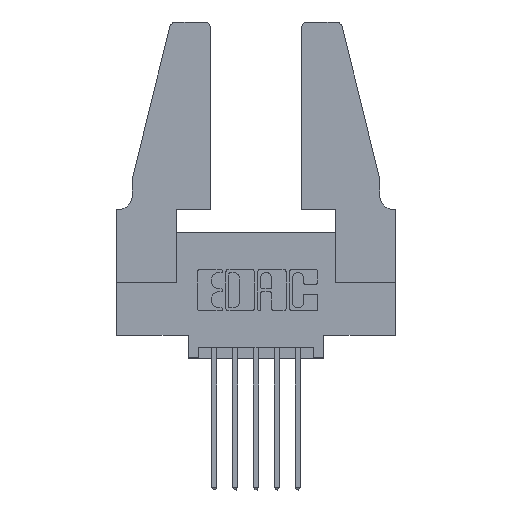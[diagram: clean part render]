
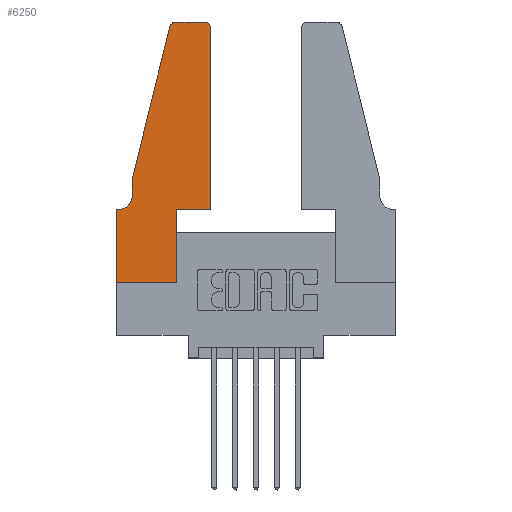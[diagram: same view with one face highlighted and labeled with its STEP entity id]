
A CAD part, top view. The second image highlights one B-rep face of the part: STEP entity #6250.
In plain terms, the highlighted planar face has unit normal (0, 0, 1).
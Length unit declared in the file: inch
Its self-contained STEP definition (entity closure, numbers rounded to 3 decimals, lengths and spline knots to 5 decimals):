
#84 = VERTEX_POINT ( 'NONE', #4923 ) ;
#313 = AXIS2_PLACEMENT_3D ( 'NONE', #5405, #5387, #5365 ) ;
#339 = VERTEX_POINT ( 'NONE', #9902 ) ;
#358 = LINE ( 'NONE', #2017, #2889 ) ;
#448 = EDGE_CURVE ( 'NONE', #6199, #8595, #9593, .T. ) ;
#531 = VECTOR ( 'NONE', #8886, 39.37008 ) ;
#560 = VERTEX_POINT ( 'NONE', #7360 ) ;
#575 = CARTESIAN_POINT ( 'NONE',  ( 0.2865, 0.35, 0.37 ) ) ;
#1094 = ORIENTED_EDGE ( 'NONE', *, *, #6711, .T. ) ;
#1309 = CIRCLE ( 'NONE', #10047, 0.03 ) ;
#1563 = ORIENTED_EDGE ( 'NONE', *, *, #6059, .T. ) ;
#1564 = VECTOR ( 'NONE', #9132, 39.37008 ) ;
#1582 = VERTEX_POINT ( 'NONE', #6077 ) ;
#1892 = DIRECTION ( 'NONE',  ( 1., 0., 0. ) ) ;
#1942 = CARTESIAN_POINT ( 'NONE',  ( 0.0755, 0.42, 0.37 ) ) ;
#2004 = CARTESIAN_POINT ( 'NONE',  ( 0., 0., 0.37 ) ) ;
#2017 = CARTESIAN_POINT ( 'NONE',  ( 0.4505, 0.35, 0.37 ) ) ;
#2124 = EDGE_CURVE ( 'NONE', #5980, #8795, #1309, .T. ) ;
#2289 = EDGE_CURVE ( 'NONE', #3363, #339, #2369, .T. ) ;
#2318 = ORIENTED_EDGE ( 'NONE', *, *, #6033, .T. ) ;
#2356 = CARTESIAN_POINT ( 'NONE',  ( 0.284, 1.22, 0.37 ) ) ;
#2369 = CIRCLE ( 'NONE', #3097, 0.07 ) ;
#2541 = DIRECTION ( 'NONE',  ( -1., 0., 0. ) ) ;
#2886 = CARTESIAN_POINT ( 'NONE',  ( 0.4505, 0.35, 0.37 ) ) ;
#2889 = VECTOR ( 'NONE', #1892, 39.37008 ) ;
#3066 = LINE ( 'NONE', #2004, #531 ) ;
#3097 = AXIS2_PLACEMENT_3D ( 'NONE', #7917, #4808, #3825 ) ;
#3243 = CARTESIAN_POINT ( 'NONE',  ( 0.0755, 0.5, 0.37 ) ) ;
#3301 = DIRECTION ( 'NONE',  ( 0., -1., 0. ) ) ;
#3363 = VERTEX_POINT ( 'NONE', #1942 ) ;
#3635 = CARTESIAN_POINT ( 'NONE',  ( 0.4505, 1.22, 0.37 ) ) ;
#3825 = DIRECTION ( 'NONE',  ( -1., 0., 0. ) ) ;
#3929 = VECTOR ( 'NONE', #4393, 39.37008 ) ;
#4336 = VECTOR ( 'NONE', #5731, 39.37008 ) ;
#4392 = DIRECTION ( 'NONE',  ( 1., 0., 0. ) ) ;
#4393 = DIRECTION ( 'NONE',  ( 0., -1., 0. ) ) ;
#4451 = ORIENTED_EDGE ( 'NONE', *, *, #4783, .T. ) ;
#4484 = ORIENTED_EDGE ( 'NONE', *, *, #448, .T. ) ;
#4754 = CARTESIAN_POINT ( 'NONE',  ( 0.2865, 0.35, 0.37 ) ) ;
#4783 = EDGE_CURVE ( 'NONE', #10551, #3363, #10555, .T. ) ;
#4808 = DIRECTION ( 'NONE',  ( 0., 0., -1. ) ) ;
#4923 = CARTESIAN_POINT ( 'NONE',  ( 0.4505, 0.35, 0.37 ) ) ;
#5096 = CARTESIAN_POINT ( 'NONE',  ( 0., 0., 0.37 ) ) ;
#5116 = VERTEX_POINT ( 'NONE', #3635 ) ;
#5298 = VECTOR ( 'NONE', #6307, 39.37008 ) ;
#5364 = PLANE ( 'NONE',  #10744 ) ;
#5365 = DIRECTION ( 'NONE',  ( 1., 0., 0. ) ) ;
#5387 = DIRECTION ( 'NONE',  ( 0., 0., 1. ) ) ;
#5405 = CARTESIAN_POINT ( 'NONE',  ( 0.4205, 1.22, 0.37 ) ) ;
#5731 = DIRECTION ( 'NONE',  ( 0., 1., 0. ) ) ;
#5738 = LINE ( 'NONE', #6946, #9743 ) ;
#5859 = DIRECTION ( 'NONE',  ( 0., 0., 1. ) ) ;
#5888 = CARTESIAN_POINT ( 'NONE',  ( 0., 0.35, 0.37 ) ) ;
#5900 = CARTESIAN_POINT ( 'NONE',  ( 0.0755, 0.35, 0.37 ) ) ;
#5980 = VERTEX_POINT ( 'NONE', #8093 ) ;
#6033 = EDGE_CURVE ( 'NONE', #8795, #10551, #9753, .T. ) ;
#6059 = EDGE_CURVE ( 'NONE', #5116, #6135, #7376, .T. ) ;
#6077 = CARTESIAN_POINT ( 'NONE',  ( 0., 0.35, 0.37 ) ) ;
#6083 = ORIENTED_EDGE ( 'NONE', *, *, #9119, .T. ) ;
#6109 = CARTESIAN_POINT ( 'NONE',  ( 0.4205, 1.25, 0.37 ) ) ;
#6117 = LINE ( 'NONE', #5096, #10153 ) ;
#6135 = VERTEX_POINT ( 'NONE', #6109 ) ;
#6199 = VERTEX_POINT ( 'NONE', #6965 ) ;
#6250 = ADVANCED_FACE ( 'NONE', ( #7728 ), #5364, .T. ) ;
#6307 = DIRECTION ( 'NONE',  ( 0., 1., 0. ) ) ;
#6541 = EDGE_LOOP ( 'NONE', ( #11154, #7040, #2318, #4451, #8522, #6083, #7369, #8906, #4484, #1094, #9809, #1563 ) ) ;
#6605 = EDGE_CURVE ( 'NONE', #84, #5116, #8477, .T. ) ;
#6711 = EDGE_CURVE ( 'NONE', #8595, #84, #358, .T. ) ;
#6946 = CARTESIAN_POINT ( 'NONE',  ( 0.2605, 1.25, 0.37 ) ) ;
#6965 = CARTESIAN_POINT ( 'NONE',  ( 0.2865, 0., 0.37 ) ) ;
#7040 = ORIENTED_EDGE ( 'NONE', *, *, #2124, .T. ) ;
#7046 = DIRECTION ( 'NONE',  ( 1., 0., 0. ) ) ;
#7360 = CARTESIAN_POINT ( 'NONE',  ( 0., 0., 0.37 ) ) ;
#7369 = ORIENTED_EDGE ( 'NONE', *, *, #9134, .T. ) ;
#7376 = CIRCLE ( 'NONE', #313, 0.03 ) ;
#7728 = FACE_OUTER_BOUND ( 'NONE', #6541, .T. ) ;
#7917 = CARTESIAN_POINT ( 'NONE',  ( 0.0055, 0.42, 0.37 ) ) ;
#7959 = CARTESIAN_POINT ( 'NONE',  ( 0.25487, 1.22718, 0.37 ) ) ;
#8093 = CARTESIAN_POINT ( 'NONE',  ( 0.284, 1.25, 0.37 ) ) ;
#8477 = LINE ( 'NONE', #2886, #4336 ) ;
#8522 = ORIENTED_EDGE ( 'NONE', *, *, #2289, .T. ) ;
#8595 = VERTEX_POINT ( 'NONE', #575 ) ;
#8795 = VERTEX_POINT ( 'NONE', #7959 ) ;
#8886 = DIRECTION ( 'NONE',  ( 1., 0., 0. ) ) ;
#8906 = ORIENTED_EDGE ( 'NONE', *, *, #10097, .T. ) ;
#9119 = EDGE_CURVE ( 'NONE', #339, #1582, #10929, .T. ) ;
#9132 = DIRECTION ( 'NONE',  ( -1., 0., 0. ) ) ;
#9134 = EDGE_CURVE ( 'NONE', #1582, #560, #6117, .T. ) ;
#9303 = CARTESIAN_POINT ( 'NONE',  ( 0.0755, 0.5, 0.37 ) ) ;
#9312 = DIRECTION ( 'NONE',  ( -0.239, -0.971, 0. ) ) ;
#9504 = VECTOR ( 'NONE', #9312, 39.37008 ) ;
#9593 = LINE ( 'NONE', #4754, #5298 ) ;
#9743 = VECTOR ( 'NONE', #2541, 39.37008 ) ;
#9753 = LINE ( 'NONE', #9303, #9504 ) ;
#9784 = EDGE_CURVE ( 'NONE', #6135, #5980, #5738, .T. ) ;
#9809 = ORIENTED_EDGE ( 'NONE', *, *, #6605, .T. ) ;
#9902 = CARTESIAN_POINT ( 'NONE',  ( 0.0055, 0.35, 0.37 ) ) ;
#10047 = AXIS2_PLACEMENT_3D ( 'NONE', #2356, #10688, #7046 ) ;
#10097 = EDGE_CURVE ( 'NONE', #560, #6199, #3066, .T. ) ;
#10153 = VECTOR ( 'NONE', #3301, 39.37008 ) ;
#10551 = VERTEX_POINT ( 'NONE', #10639 ) ;
#10555 = LINE ( 'NONE', #3243, #3929 ) ;
#10639 = CARTESIAN_POINT ( 'NONE',  ( 0.0755, 0.5, 0.37 ) ) ;
#10688 = DIRECTION ( 'NONE',  ( 0., 0., 1. ) ) ;
#10744 = AXIS2_PLACEMENT_3D ( 'NONE', #5888, #5859, #4392 ) ;
#10929 = LINE ( 'NONE', #5900, #1564 ) ;
#11154 = ORIENTED_EDGE ( 'NONE', *, *, #9784, .T. ) ;
